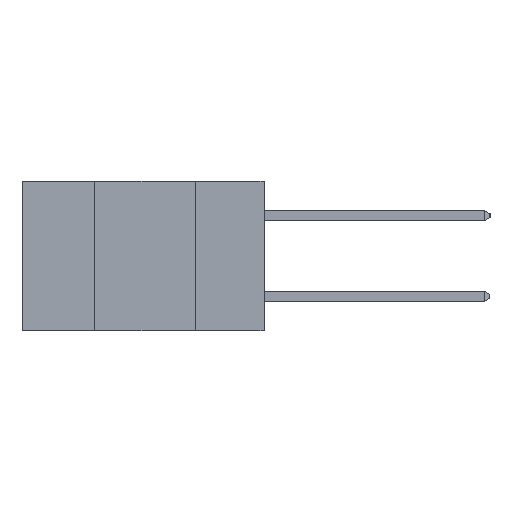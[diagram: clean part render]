
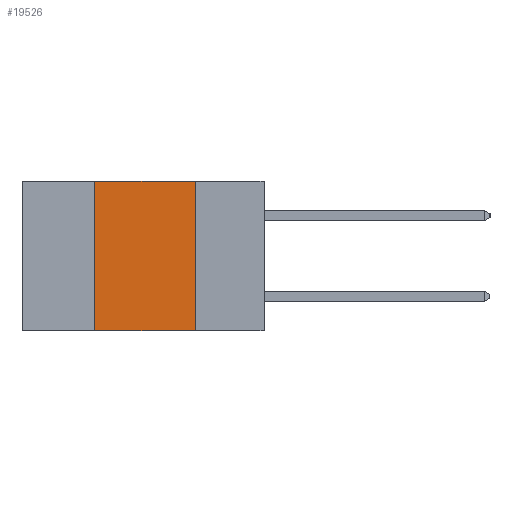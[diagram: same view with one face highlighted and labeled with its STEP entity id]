
A CAD part, left-side view. The second image highlights one B-rep face of the part: STEP entity #19526.
In plain terms, the highlighted planar face has unit normal (-1, 0, 0).
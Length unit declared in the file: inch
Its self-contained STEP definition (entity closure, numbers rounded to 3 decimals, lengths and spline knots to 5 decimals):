
#109 = VERTEX_POINT ( 'NONE', #1939 ) ;
#175 = AXIS2_PLACEMENT_3D ( 'NONE', #13283, #2808, #14997 ) ;
#546 = LINE ( 'NONE', #9961, #14047 ) ;
#963 = PLANE ( 'NONE',  #175 ) ;
#1939 = CARTESIAN_POINT ( 'NONE',  ( 0., 0.42, -0.37 ) ) ;
#2808 = DIRECTION ( 'NONE',  ( 1., 0., 0. ) ) ;
#3865 = DIRECTION ( 'NONE',  ( 0., -1., 0. ) ) ;
#5440 = CARTESIAN_POINT ( 'NONE',  ( 0., 0.6, 0. ) ) ;
#6167 = VERTEX_POINT ( 'NONE', #10361 ) ;
#7307 = CARTESIAN_POINT ( 'NONE',  ( 0., 0.6, -0.37 ) ) ;
#8425 = EDGE_CURVE ( 'NONE', #17602, #6167, #546, .T. ) ;
#8837 = CARTESIAN_POINT ( 'NONE',  ( 0., 0.17, 0. ) ) ;
#9608 = EDGE_CURVE ( 'NONE', #109, #14848, #13170, .T. ) ;
#9961 = CARTESIAN_POINT ( 'NONE',  ( 0., 0.17, -0.37 ) ) ;
#9964 = DIRECTION ( 'NONE',  ( 0., 0., -1. ) ) ;
#10361 = CARTESIAN_POINT ( 'NONE',  ( 0., 0.17, -0.37 ) ) ;
#10484 = ORIENTED_EDGE ( 'NONE', *, *, #8425, .F. ) ;
#10667 = ORIENTED_EDGE ( 'NONE', *, *, #20424, .F. ) ;
#11805 = ORIENTED_EDGE ( 'NONE', *, *, #22319, .T. ) ;
#13170 = LINE ( 'NONE', #19279, #18316 ) ;
#13209 = LINE ( 'NONE', #5440, #21273 ) ;
#13283 = CARTESIAN_POINT ( 'NONE',  ( 0., 0.6, 0. ) ) ;
#13389 = LINE ( 'NONE', #7307, #21959 ) ;
#14047 = VECTOR ( 'NONE', #9964, 39.37008 ) ;
#14848 = VERTEX_POINT ( 'NONE', #22386 ) ;
#14997 = DIRECTION ( 'NONE',  ( 0., 0., -1. ) ) ;
#17545 = DIRECTION ( 'NONE',  ( 0., -1., 0. ) ) ;
#17602 = VERTEX_POINT ( 'NONE', #8837 ) ;
#17956 = EDGE_LOOP ( 'NONE', ( #10484, #10667, #20959, #11805 ) ) ;
#18316 = VECTOR ( 'NONE', #18999, 39.37008 ) ;
#18999 = DIRECTION ( 'NONE',  ( 0., 0., 1. ) ) ;
#19279 = CARTESIAN_POINT ( 'NONE',  ( 0., 0.42, -0.37 ) ) ;
#19526 = ADVANCED_FACE ( 'NONE', ( #21313 ), #963, .F. ) ;
#20424 = EDGE_CURVE ( 'NONE', #14848, #17602, #13209, .T. ) ;
#20959 = ORIENTED_EDGE ( 'NONE', *, *, #9608, .F. ) ;
#21273 = VECTOR ( 'NONE', #17545, 39.37008 ) ;
#21313 = FACE_OUTER_BOUND ( 'NONE', #17956, .T. ) ;
#21959 = VECTOR ( 'NONE', #3865, 39.37008 ) ;
#22319 = EDGE_CURVE ( 'NONE', #109, #6167, #13389, .T. ) ;
#22386 = CARTESIAN_POINT ( 'NONE',  ( 0., 0.42, 0. ) ) ;
